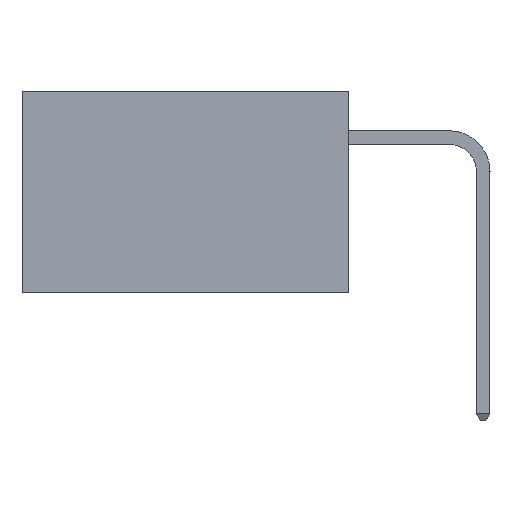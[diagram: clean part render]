
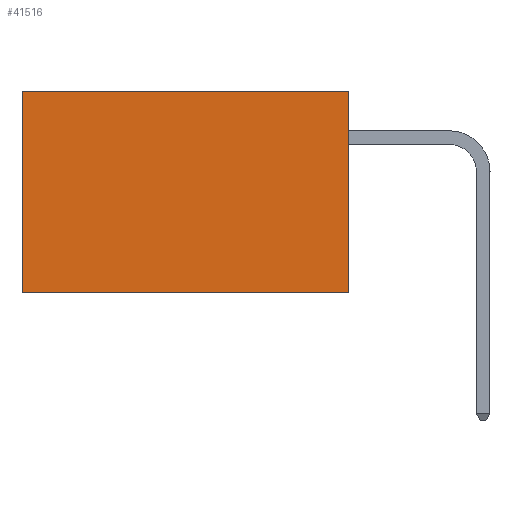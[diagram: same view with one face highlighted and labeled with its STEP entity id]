
A CAD part, left-side view. The second image highlights one B-rep face of the part: STEP entity #41516.
In plain terms, the highlighted planar face has unit normal (-1, 0, 0).
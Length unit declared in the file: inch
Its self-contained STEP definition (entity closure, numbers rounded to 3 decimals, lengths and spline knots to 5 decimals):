
#1182 = EDGE_CURVE ( 'NONE', #7952, #10154, #4007, .T. ) ;
#1204 = VECTOR ( 'NONE', #7767, 39.37008 ) ;
#3478 = CARTESIAN_POINT ( 'NONE',  ( 0.2875, 0., 0. ) ) ;
#4007 = LINE ( 'NONE', #16295, #40371 ) ;
#6136 = VECTOR ( 'NONE', #19013, 39.37008 ) ;
#7767 = DIRECTION ( 'NONE',  ( 0., 1., 0. ) ) ;
#7952 = VERTEX_POINT ( 'NONE', #21856 ) ;
#8806 = ORIENTED_EDGE ( 'NONE', *, *, #30577, .F. ) ;
#9100 = EDGE_CURVE ( 'NONE', #30566, #41632, #29325, .T. ) ;
#9881 = PLANE ( 'NONE',  #29588 ) ;
#10154 = VERTEX_POINT ( 'NONE', #20814 ) ;
#10494 = CARTESIAN_POINT ( 'NONE',  ( 0.2875, 0.6, 0. ) ) ;
#13460 = DIRECTION ( 'NONE',  ( 1., 0., 0. ) ) ;
#14741 = LINE ( 'NONE', #29235, #32345 ) ;
#15185 = ORIENTED_EDGE ( 'NONE', *, *, #1182, .F. ) ;
#15543 = EDGE_CURVE ( 'NONE', #41632, #10154, #24867, .T. ) ;
#16295 = CARTESIAN_POINT ( 'NONE',  ( 0.2875, 0., -0.37 ) ) ;
#17740 = DIRECTION ( 'NONE',  ( 0., 0., -1. ) ) ;
#18990 = ORIENTED_EDGE ( 'NONE', *, *, #15543, .T. ) ;
#19013 = DIRECTION ( 'NONE',  ( 0., 0., -1. ) ) ;
#20814 = CARTESIAN_POINT ( 'NONE',  ( 0.2875, 0.6, -0.37 ) ) ;
#21819 = CARTESIAN_POINT ( 'NONE',  ( 0.2875, 0., 0. ) ) ;
#21856 = CARTESIAN_POINT ( 'NONE',  ( 0.2875, 0., -0.37 ) ) ;
#23727 = ORIENTED_EDGE ( 'NONE', *, *, #9100, .T. ) ;
#23901 = CARTESIAN_POINT ( 'NONE',  ( 0.2875, 0., 0. ) ) ;
#24841 = FACE_OUTER_BOUND ( 'NONE', #31465, .T. ) ;
#24867 = LINE ( 'NONE', #43520, #6136 ) ;
#29235 = CARTESIAN_POINT ( 'NONE',  ( 0.2875, 0., 0. ) ) ;
#29267 = DIRECTION ( 'NONE',  ( 0., 1., 0. ) ) ;
#29325 = LINE ( 'NONE', #21819, #1204 ) ;
#29588 = AXIS2_PLACEMENT_3D ( 'NONE', #23901, #13460, #38001 ) ;
#30566 = VERTEX_POINT ( 'NONE', #3478 ) ;
#30577 = EDGE_CURVE ( 'NONE', #30566, #7952, #14741, .T. ) ;
#31465 = EDGE_LOOP ( 'NONE', ( #18990, #15185, #8806, #23727 ) ) ;
#32345 = VECTOR ( 'NONE', #17740, 39.37008 ) ;
#38001 = DIRECTION ( 'NONE',  ( 0., 0., -1. ) ) ;
#40371 = VECTOR ( 'NONE', #29267, 39.37008 ) ;
#41516 = ADVANCED_FACE ( 'NONE', ( #24841 ), #9881, .F. ) ;
#41632 = VERTEX_POINT ( 'NONE', #10494 ) ;
#43520 = CARTESIAN_POINT ( 'NONE',  ( 0.2875, 0.6, 0. ) ) ;
